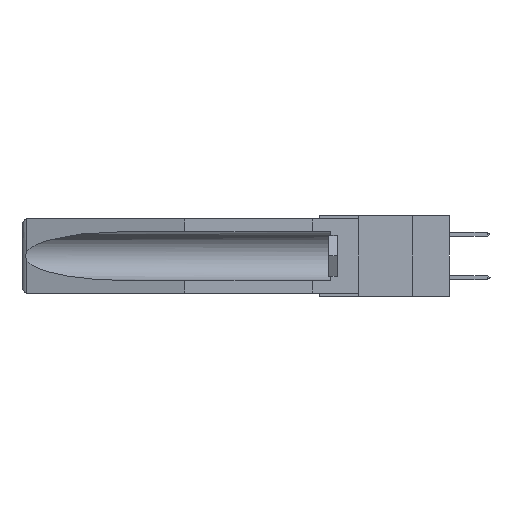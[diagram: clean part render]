
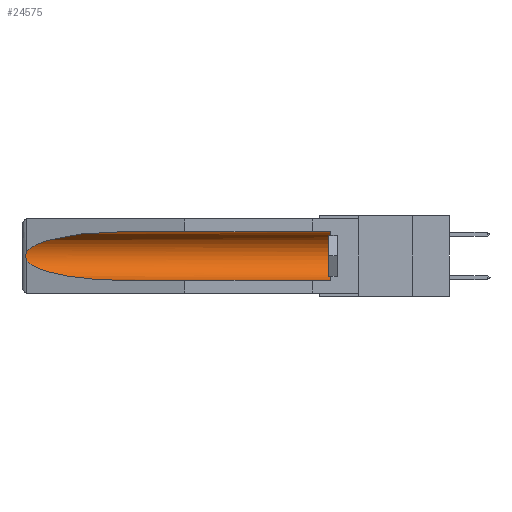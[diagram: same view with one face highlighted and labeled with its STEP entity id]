
A CAD part, left-side view. The second image highlights one B-rep face of the part: STEP entity #24575.
In plain terms, the highlighted cylindrical face has radius 2.857 mm (diameter 5.715 mm), a partial arc.
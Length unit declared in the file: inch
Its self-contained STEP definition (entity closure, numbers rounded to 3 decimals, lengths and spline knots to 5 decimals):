
#174 = CARTESIAN_POINT ( 'NONE',  ( 0.155, -0.30754, -0.284 ) ) ;
#806 = CARTESIAN_POINT ( 'NONE',  ( 0.155, 1.07973, -0.059 ) ) ;
#1121 = EDGE_CURVE ( 'NONE', #8546, #19960, #23039, .T. ) ;
#1377 = AXIS2_PLACEMENT_3D ( 'NONE', #10827, #6899, #23386 ) ;
#3258 = CARTESIAN_POINT ( 'NONE',  ( 0.25451, 1.48313, -0.09465 ) ) ;
#3956 = ORIENTED_EDGE ( 'NONE', *, *, #10629, .T. ) ;
#3973 = VERTEX_POINT ( 'NONE', #6976 ) ;
#4306 = CARTESIAN_POINT ( 'NONE',  ( 0.155, 1.07973, -0.284 ) ) ;
#4384 = CARTESIAN_POINT ( 'NONE',  ( 0.25451, 1.48313, -0.24835 ) ) ;
#6288 = CARTESIAN_POINT ( 'NONE',  ( 0.2673, 1.53269, -0.17917 ) ) ;
#6888 = FACE_OUTER_BOUND ( 'NONE', #25300, .T. ) ;
#6899 = DIRECTION ( 'NONE',  ( 0., -1., 0. ) ) ;
#6976 = CARTESIAN_POINT ( 'NONE',  ( 0.26537, 1.52718, -0.19328 ) ) ;
#7125 = CARTESIAN_POINT ( 'NONE',  ( 0.155, -0.30754, -0.059 ) ) ;
#8391 = CARTESIAN_POINT ( 'NONE',  ( 0.26597, 1.5296, -0.19026 ) ) ;
#8545 = CARTESIAN_POINT ( 'NONE',  ( 0.21114, 1.30732, -0.284 ) ) ;
#8546 = VERTEX_POINT ( 'NONE', #11329 ) ;
#8572 = ORIENTED_EDGE ( 'NONE', *, *, #10590, .T. ) ;
#10017 = ORIENTED_EDGE ( 'NONE', *, *, #18742, .T. ) ;
#10126 = CARTESIAN_POINT ( 'NONE',  ( 0.26597, 1.52961, -0.15275 ) ) ;
#10320 = CARTESIAN_POINT ( 'NONE',  ( 0.26654, 1.53092, -0.15636 ) ) ;
#10474 = CARTESIAN_POINT ( 'NONE',  ( 0.155, 0.126, -0.284 ) ) ;
#10568 = CARTESIAN_POINT ( 'NONE',  ( 0.26537, 1.52718, -0.19328 ) ) ;
#10590 = EDGE_CURVE ( 'NONE', #3973, #23414, #25505, .T. ) ;
#10629 = EDGE_CURVE ( 'NONE', #24370, #8546, #17660, .T. ) ;
#10664 = CARTESIAN_POINT ( 'NONE',  ( 0.155, 1.07973, -0.284 ) ) ;
#10827 = CARTESIAN_POINT ( 'NONE',  ( 0.155, 0.126, -0.1715 ) ) ;
#11070 =( BOUNDED_CURVE ( )  B_SPLINE_CURVE ( 3, ( #13556, #15688, #3258, #25865 ),
 .UNSPECIFIED., .F., .F. ) 
 B_SPLINE_CURVE_WITH_KNOTS ( ( 4, 4 ),
 ( 4.71239, 6.08839 ),
 .UNSPECIFIED. ) 
 CURVE ( )  GEOMETRIC_REPRESENTATION_ITEM ( )  RATIONAL_B_SPLINE_CURVE ( ( 1., 0.848, 0.848, 1. ) ) 
 REPRESENTATION_ITEM ( '' )  );
#11250 = DIRECTION ( 'NONE',  ( 0., 0., 1. ) ) ;
#11329 = CARTESIAN_POINT ( 'NONE',  ( 0.155, 0.126, -0.059 ) ) ;
#11417 = ORIENTED_EDGE ( 'NONE', *, *, #15376, .T. ) ;
#11910 = B_SPLINE_CURVE_WITH_KNOTS ( 'NONE', 3,
 ( #12294, #10126, #10320, #26497, #20990, #24869, #6288, #20810, #8391, #12733 ),
 .UNSPECIFIED., .F., .F.,
 ( 4, 2, 2, 2, 4 ),
 ( 0., 0.00029, 0.00058, 0.00087, 0.00117 ),
 .UNSPECIFIED. ) ;
#12294 = CARTESIAN_POINT ( 'NONE',  ( 0.26537, 1.52718, -0.14972 ) ) ;
#12733 = CARTESIAN_POINT ( 'NONE',  ( 0.26537, 1.52718, -0.19328 ) ) ;
#13135 = VECTOR ( 'NONE', #19572, 39.37008 ) ;
#13556 = CARTESIAN_POINT ( 'NONE',  ( 0.155, 1.07973, -0.059 ) ) ;
#15376 = EDGE_CURVE ( 'NONE', #19960, #22836, #11070, .T. ) ;
#15688 = CARTESIAN_POINT ( 'NONE',  ( 0.21114, 1.30732, -0.059 ) ) ;
#17113 = ORIENTED_EDGE ( 'NONE', *, *, #1121, .T. ) ;
#17221 = CYLINDRICAL_SURFACE ( 'NONE', #25006, 0.1125 ) ;
#17621 = DIRECTION ( 'NONE',  ( 0., 1., 0. ) ) ;
#17660 = CIRCLE ( 'NONE', #1377, 0.1125 ) ;
#17712 = CARTESIAN_POINT ( 'NONE',  ( 0.155, -0.30754, -0.1715 ) ) ;
#18742 = EDGE_CURVE ( 'NONE', #22836, #3973, #11910, .T. ) ;
#19374 = CARTESIAN_POINT ( 'NONE',  ( 0.26537, 1.52718, -0.14972 ) ) ;
#19572 = DIRECTION ( 'NONE',  ( 0., 1., 0. ) ) ;
#19684 = DIRECTION ( 'NONE',  ( 0., 1., 0. ) ) ;
#19960 = VERTEX_POINT ( 'NONE', #806 ) ;
#20810 = CARTESIAN_POINT ( 'NONE',  ( 0.26655, 1.53094, -0.18657 ) ) ;
#20990 = CARTESIAN_POINT ( 'NONE',  ( 0.2675, 1.53308, -0.16763 ) ) ;
#21089 = VECTOR ( 'NONE', #19684, 39.37008 ) ;
#21482 = ORIENTED_EDGE ( 'NONE', *, *, #22587, .F. ) ;
#22587 = EDGE_CURVE ( 'NONE', #24370, #23414, #22844, .T. ) ;
#22836 = VERTEX_POINT ( 'NONE', #19374 ) ;
#22844 = LINE ( 'NONE', #174, #13135 ) ;
#23039 = LINE ( 'NONE', #7125, #21089 ) ;
#23386 = DIRECTION ( 'NONE',  ( 0., 0., 1. ) ) ;
#23414 = VERTEX_POINT ( 'NONE', #4306 ) ;
#24370 = VERTEX_POINT ( 'NONE', #10474 ) ;
#24575 = ADVANCED_FACE ( 'NONE', ( #6888 ), #17221, .F. ) ;
#24869 = CARTESIAN_POINT ( 'NONE',  ( 0.2675, 1.53308, -0.17534 ) ) ;
#25006 = AXIS2_PLACEMENT_3D ( 'NONE', #17712, #17621, #11250 ) ;
#25300 = EDGE_LOOP ( 'NONE', ( #11417, #10017, #8572, #21482, #3956, #17113 ) ) ;
#25505 =( BOUNDED_CURVE ( )  B_SPLINE_CURVE ( 3, ( #10568, #4384, #8545, #10664 ),
 .UNSPECIFIED., .F., .T. ) 
 B_SPLINE_CURVE_WITH_KNOTS ( ( 4, 4 ),
 ( 0.1948, 1.5708 ),
 .UNSPECIFIED. ) 
 CURVE ( )  GEOMETRIC_REPRESENTATION_ITEM ( )  RATIONAL_B_SPLINE_CURVE ( ( 1., 0.848, 0.848, 1. ) ) 
 REPRESENTATION_ITEM ( '' )  );
#25865 = CARTESIAN_POINT ( 'NONE',  ( 0.26537, 1.52718, -0.14972 ) ) ;
#26497 = CARTESIAN_POINT ( 'NONE',  ( 0.2673, 1.5327, -0.16383 ) ) ;
